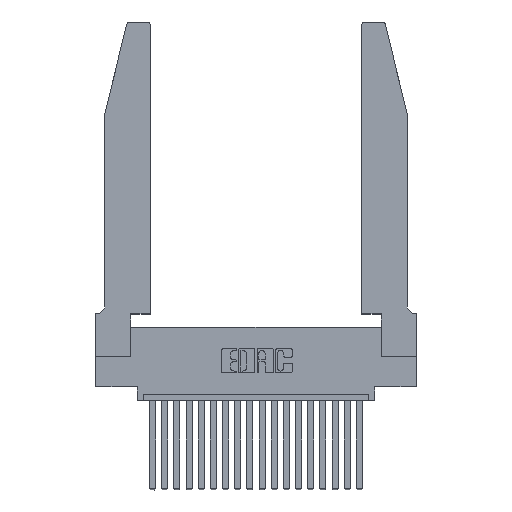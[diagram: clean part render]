
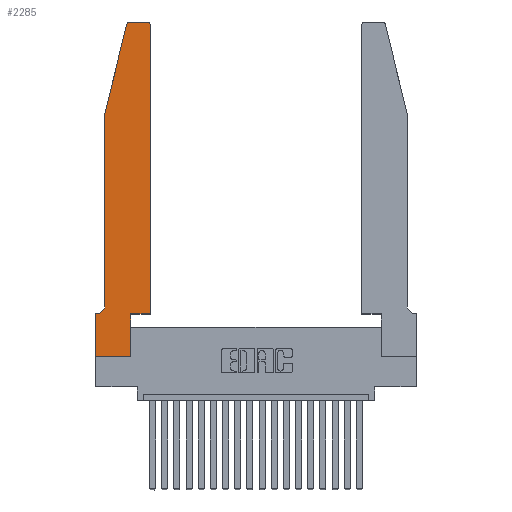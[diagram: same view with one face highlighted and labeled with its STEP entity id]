
A CAD part, top view. The second image highlights one B-rep face of the part: STEP entity #2285.
In plain terms, the highlighted planar face has unit normal (0, 0, 1).
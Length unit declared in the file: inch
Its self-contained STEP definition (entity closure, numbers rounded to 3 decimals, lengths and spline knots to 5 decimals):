
#103 = VECTOR ( 'NONE', #19468, 39.37008 ) ;
#104 = EDGE_CURVE ( 'NONE', #7201, #11729, #14388, .T. ) ;
#170 = CARTESIAN_POINT ( 'NONE',  ( 0.4505, 0.35, 0.37 ) ) ;
#210 = CARTESIAN_POINT ( 'NONE',  ( 0.4505, 0.35, 0.37 ) ) ;
#293 = ORIENTED_EDGE ( 'NONE', *, *, #17287, .T. ) ;
#729 = VERTEX_POINT ( 'NONE', #12674 ) ;
#2084 = PLANE ( 'NONE',  #15751 ) ;
#2285 = ADVANCED_FACE ( 'NONE', ( #3900 ), #2084, .T. ) ;
#2288 = VERTEX_POINT ( 'NONE', #18692 ) ;
#2352 = VECTOR ( 'NONE', #6625, 39.37008 ) ;
#2370 = CIRCLE ( 'NONE', #13951, 0.03 ) ;
#2961 = DIRECTION ( 'NONE',  ( -1., 0., 0. ) ) ;
#3010 = ORIENTED_EDGE ( 'NONE', *, *, #18849, .T. ) ;
#3142 = VECTOR ( 'NONE', #10862, 39.37008 ) ;
#3407 = VERTEX_POINT ( 'NONE', #16377 ) ;
#3642 = EDGE_CURVE ( 'NONE', #11729, #21469, #16866, .T. ) ;
#3671 = VECTOR ( 'NONE', #6538, 39.37008 ) ;
#3689 = DIRECTION ( 'NONE',  ( 1., 0., 0. ) ) ;
#3799 = ORIENTED_EDGE ( 'NONE', *, *, #18956, .T. ) ;
#3900 = FACE_OUTER_BOUND ( 'NONE', #6621, .T. ) ;
#3906 = VECTOR ( 'NONE', #4001, 39.37008 ) ;
#4001 = DIRECTION ( 'NONE',  ( 0., 1., 0. ) ) ;
#4227 = VERTEX_POINT ( 'NONE', #10139 ) ;
#4398 = VERTEX_POINT ( 'NONE', #9114 ) ;
#4673 = LINE ( 'NONE', #4967, #2352 ) ;
#4775 = DIRECTION ( 'NONE',  ( 0., 0., -1. ) ) ;
#4967 = CARTESIAN_POINT ( 'NONE',  ( 0.2605, 2.75, 0.37 ) ) ;
#5041 = CARTESIAN_POINT ( 'NONE',  ( 0.0755, 2., 0.37 ) ) ;
#5295 = DIRECTION ( 'NONE',  ( 1., 0., 0. ) ) ;
#5437 = LINE ( 'NONE', #13797, #20999 ) ;
#5589 = CARTESIAN_POINT ( 'NONE',  ( 0.2865, 0.35, 0.37 ) ) ;
#5969 = VERTEX_POINT ( 'NONE', #12913 ) ;
#6140 = EDGE_CURVE ( 'NONE', #2288, #9762, #2370, .T. ) ;
#6210 = VERTEX_POINT ( 'NONE', #210 ) ;
#6260 = LINE ( 'NONE', #20883, #3142 ) ;
#6305 = VECTOR ( 'NONE', #19609, 39.37008 ) ;
#6404 = CARTESIAN_POINT ( 'NONE',  ( 0.4505, 0.35, 0.37 ) ) ;
#6538 = DIRECTION ( 'NONE',  ( 1., 0., 0. ) ) ;
#6621 = EDGE_LOOP ( 'NONE', ( #12066, #293, #18256, #18257, #3799, #21447, #3010, #20715, #15963, #11748, #11390, #17476 ) ) ;
#6625 = DIRECTION ( 'NONE',  ( -1., 0., 0. ) ) ;
#6727 = DIRECTION ( 'NONE',  ( -0.239, -0.971, 0. ) ) ;
#6734 = EDGE_CURVE ( 'NONE', #9762, #4227, #4673, .T. ) ;
#6985 = EDGE_CURVE ( 'NONE', #19522, #3407, #8309, .T. ) ;
#7201 = VERTEX_POINT ( 'NONE', #8409 ) ;
#7375 = EDGE_CURVE ( 'NONE', #5969, #19522, #5437, .T. ) ;
#7393 = CARTESIAN_POINT ( 'NONE',  ( 0.284, 2.72, 0.37 ) ) ;
#7713 = AXIS2_PLACEMENT_3D ( 'NONE', #7393, #8987, #13883 ) ;
#7714 = CARTESIAN_POINT ( 'NONE',  ( 0.2865, 0., 0.37 ) ) ;
#7997 = VECTOR ( 'NONE', #11837, 39.37008 ) ;
#8051 = LINE ( 'NONE', #170, #3671 ) ;
#8275 = CARTESIAN_POINT ( 'NONE',  ( 0.4205, 2.75, 0.37 ) ) ;
#8309 = LINE ( 'NONE', #5589, #3906 ) ;
#8379 = VECTOR ( 'NONE', #6727, 39.37008 ) ;
#8409 = CARTESIAN_POINT ( 'NONE',  ( 0.25487, 2.72718, 0.37 ) ) ;
#8682 = DIRECTION ( 'NONE',  ( 0., 0., 1. ) ) ;
#8987 = DIRECTION ( 'NONE',  ( 0., 0., 1. ) ) ;
#9114 = CARTESIAN_POINT ( 'NONE',  ( 0.0055, 0.35, 0.37 ) ) ;
#9762 = VERTEX_POINT ( 'NONE', #8275 ) ;
#10139 = CARTESIAN_POINT ( 'NONE',  ( 0.284, 2.75, 0.37 ) ) ;
#10777 = EDGE_CURVE ( 'NONE', #4398, #729, #10970, .T. ) ;
#10862 = DIRECTION ( 'NONE',  ( 0., -1., 0. ) ) ;
#10911 = EDGE_CURVE ( 'NONE', #6210, #2288, #13866, .T. ) ;
#10970 = LINE ( 'NONE', #12665, #103 ) ;
#11357 = CARTESIAN_POINT ( 'NONE',  ( 0.4205, 2.72, 0.37 ) ) ;
#11390 = ORIENTED_EDGE ( 'NONE', *, *, #10911, .T. ) ;
#11729 = VERTEX_POINT ( 'NONE', #5041 ) ;
#11748 = ORIENTED_EDGE ( 'NONE', *, *, #18658, .T. ) ;
#11837 = DIRECTION ( 'NONE',  ( 0., -1., 0. ) ) ;
#12066 = ORIENTED_EDGE ( 'NONE', *, *, #6734, .T. ) ;
#12122 = CARTESIAN_POINT ( 'NONE',  ( 0.0755, 0.42, 0.37 ) ) ;
#12665 = CARTESIAN_POINT ( 'NONE',  ( 0.0755, 0.35, 0.37 ) ) ;
#12674 = CARTESIAN_POINT ( 'NONE',  ( 0., 0.35, 0.37 ) ) ;
#12913 = CARTESIAN_POINT ( 'NONE',  ( 0., 0., 0.37 ) ) ;
#13201 = CARTESIAN_POINT ( 'NONE',  ( 0.0755, 2., 0.37 ) ) ;
#13709 = CARTESIAN_POINT ( 'NONE',  ( 0., 0.35, 0.37 ) ) ;
#13797 = CARTESIAN_POINT ( 'NONE',  ( 0., 0., 0.37 ) ) ;
#13866 = LINE ( 'NONE', #6404, #6305 ) ;
#13883 = DIRECTION ( 'NONE',  ( 1., 0., 0. ) ) ;
#13951 = AXIS2_PLACEMENT_3D ( 'NONE', #11357, #18270, #14822 ) ;
#14388 = LINE ( 'NONE', #13201, #8379 ) ;
#14793 = CARTESIAN_POINT ( 'NONE',  ( 0.0755, 2., 0.37 ) ) ;
#14822 = DIRECTION ( 'NONE',  ( 1., 0., 0. ) ) ;
#15751 = AXIS2_PLACEMENT_3D ( 'NONE', #13709, #8682, #3689 ) ;
#15963 = ORIENTED_EDGE ( 'NONE', *, *, #6985, .T. ) ;
#16127 = CIRCLE ( 'NONE', #17769, 0.07 ) ;
#16377 = CARTESIAN_POINT ( 'NONE',  ( 0.2865, 0.35, 0.37 ) ) ;
#16866 = LINE ( 'NONE', #14793, #7997 ) ;
#17287 = EDGE_CURVE ( 'NONE', #4227, #7201, #20335, .T. ) ;
#17476 = ORIENTED_EDGE ( 'NONE', *, *, #6140, .T. ) ;
#17769 = AXIS2_PLACEMENT_3D ( 'NONE', #18065, #4775, #2961 ) ;
#18065 = CARTESIAN_POINT ( 'NONE',  ( 0.0055, 0.42, 0.37 ) ) ;
#18256 = ORIENTED_EDGE ( 'NONE', *, *, #104, .T. ) ;
#18257 = ORIENTED_EDGE ( 'NONE', *, *, #3642, .T. ) ;
#18270 = DIRECTION ( 'NONE',  ( 0., 0., 1. ) ) ;
#18658 = EDGE_CURVE ( 'NONE', #3407, #6210, #8051, .T. ) ;
#18692 = CARTESIAN_POINT ( 'NONE',  ( 0.4505, 2.72, 0.37 ) ) ;
#18849 = EDGE_CURVE ( 'NONE', #729, #5969, #6260, .T. ) ;
#18956 = EDGE_CURVE ( 'NONE', #21469, #4398, #16127, .T. ) ;
#19468 = DIRECTION ( 'NONE',  ( -1., 0., 0. ) ) ;
#19522 = VERTEX_POINT ( 'NONE', #7714 ) ;
#19609 = DIRECTION ( 'NONE',  ( 0., 1., 0. ) ) ;
#20335 = CIRCLE ( 'NONE', #7713, 0.03 ) ;
#20715 = ORIENTED_EDGE ( 'NONE', *, *, #7375, .T. ) ;
#20883 = CARTESIAN_POINT ( 'NONE',  ( 0., 0., 0.37 ) ) ;
#20999 = VECTOR ( 'NONE', #5295, 39.37008 ) ;
#21447 = ORIENTED_EDGE ( 'NONE', *, *, #10777, .T. ) ;
#21469 = VERTEX_POINT ( 'NONE', #12122 ) ;
